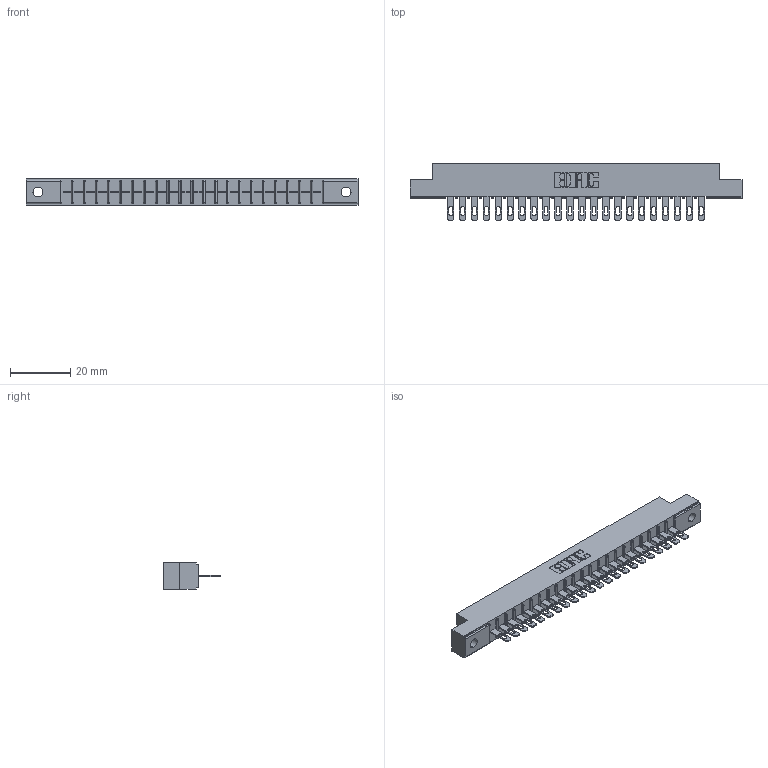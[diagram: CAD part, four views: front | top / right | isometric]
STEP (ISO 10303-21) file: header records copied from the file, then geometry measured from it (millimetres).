
FILE_DESCRIPTION (( 'STEP AP203' ), '1' );
FILE_NAME ('316-022-500-102.STEP', '2018-07-31T01:50:10', ( '' ), ( '' ), 'SwSTEP 2.0', 'SolidWorks 2016', '' );
FILE_SCHEMA (( 'CONFIG_CONTROL_DESIGN' ));
Length unit declared in the file: inch
Products named in the file (3): 306 Part_.128 Dia; 306-290-001_100; 316-022-500-102
Assembly tree (23 placements, depth 2):
  316-022-500-102
    306 Part_.128 Dia
    306-290-001_100  x22
Bounding box: 110.19 x 18.87 x 8.71 mm (x, y, z)
Volume: 7573.9 mm3; surface area: 11277.4 mm2
Topology: 23 solids, 23 shells, 1788 faces, 5046 edges, 3244 vertices
Faces by surface type: plane 1168, cylinder 532, sphere 88
Entity records: 23273 total; most frequent: CARTESIAN_POINT 3905, ORIENTED_EDGE 3868, DIRECTION 3854, EDGE_CURVE 1934, VECTOR 1500, LINE 1500, VERTEX_POINT 1228, AXIS2_PLACEMENT_3D 1177
